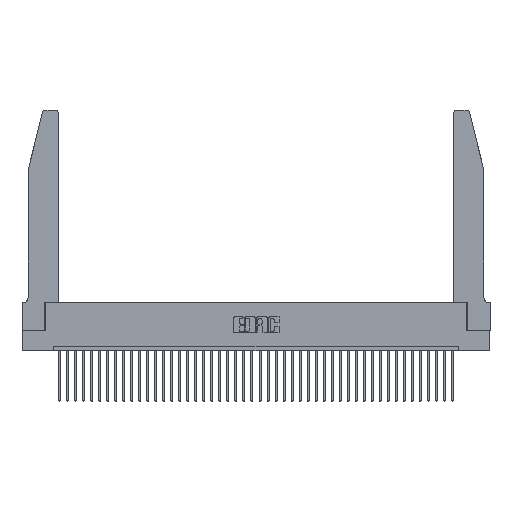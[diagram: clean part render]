
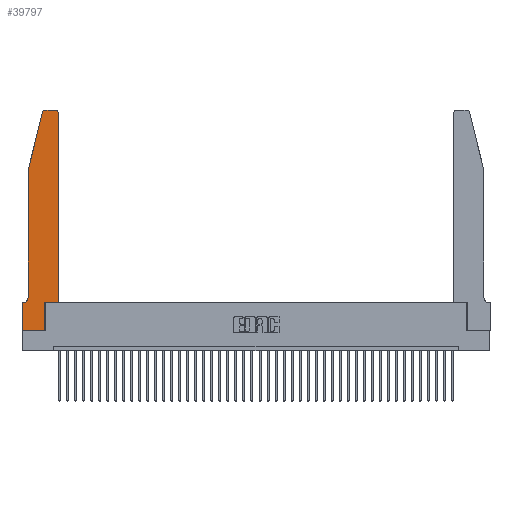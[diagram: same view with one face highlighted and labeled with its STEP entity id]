
A CAD part, top view. The second image highlights one B-rep face of the part: STEP entity #39797.
In plain terms, the highlighted planar face has unit normal (0, 0, 1).
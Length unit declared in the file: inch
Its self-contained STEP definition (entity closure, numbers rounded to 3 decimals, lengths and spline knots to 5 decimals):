
#245 = CARTESIAN_POINT ( 'NONE',  ( 0.2605, 2.75, 0.37 ) ) ;
#407 = DIRECTION ( 'NONE',  ( 0., 0., 1. ) ) ;
#1341 = EDGE_CURVE ( 'NONE', #6406, #1973, #36287, .T. ) ;
#1725 = ORIENTED_EDGE ( 'NONE', *, *, #28265, .T. ) ;
#1838 = CARTESIAN_POINT ( 'NONE',  ( 0.0755, 0.42, 0.37 ) ) ;
#1933 = VECTOR ( 'NONE', #41183, 39.37008 ) ;
#1973 = VERTEX_POINT ( 'NONE', #23858 ) ;
#3191 = VECTOR ( 'NONE', #6481, 39.37008 ) ;
#3298 = EDGE_CURVE ( 'NONE', #7035, #13448, #33613, .T. ) ;
#3389 = CIRCLE ( 'NONE', #29371, 0.07 ) ;
#3445 = DIRECTION ( 'NONE',  ( 0., -1., 0. ) ) ;
#4053 = VECTOR ( 'NONE', #23248, 39.37008 ) ;
#4185 = EDGE_CURVE ( 'NONE', #31133, #15179, #14031, .T. ) ;
#4513 = ORIENTED_EDGE ( 'NONE', *, *, #4185, .T. ) ;
#4682 = AXIS2_PLACEMENT_3D ( 'NONE', #6914, #13585, #29245 ) ;
#5447 = CARTESIAN_POINT ( 'NONE',  ( 0., 0., 0.37 ) ) ;
#5578 = EDGE_CURVE ( 'NONE', #13024, #22417, #24457, .T. ) ;
#5705 = CARTESIAN_POINT ( 'NONE',  ( 0.2865, 0.35, 0.37 ) ) ;
#5996 = CARTESIAN_POINT ( 'NONE',  ( 0.4205, 2.72, 0.37 ) ) ;
#6406 = VERTEX_POINT ( 'NONE', #21333 ) ;
#6481 = DIRECTION ( 'NONE',  ( -1., 0., 0. ) ) ;
#6540 = DIRECTION ( 'NONE',  ( 0., 1., 0. ) ) ;
#6914 = CARTESIAN_POINT ( 'NONE',  ( 0.284, 2.72, 0.37 ) ) ;
#7035 = VERTEX_POINT ( 'NONE', #37750 ) ;
#8362 = EDGE_CURVE ( 'NONE', #13448, #25497, #3389, .T. ) ;
#9171 = DIRECTION ( 'NONE',  ( 1., 0., 0. ) ) ;
#9364 = ORIENTED_EDGE ( 'NONE', *, *, #33324, .T. ) ;
#10169 = AXIS2_PLACEMENT_3D ( 'NONE', #5996, #28294, #9171 ) ;
#10204 = VECTOR ( 'NONE', #11712, 39.37008 ) ;
#10423 = VECTOR ( 'NONE', #3445, 39.37008 ) ;
#11712 = DIRECTION ( 'NONE',  ( -1., 0., 0. ) ) ;
#11817 = AXIS2_PLACEMENT_3D ( 'NONE', #38671, #407, #22762 ) ;
#12110 = LINE ( 'NONE', #245, #3191 ) ;
#12768 = ORIENTED_EDGE ( 'NONE', *, *, #27010, .T. ) ;
#13024 = VERTEX_POINT ( 'NONE', #29692 ) ;
#13448 = VERTEX_POINT ( 'NONE', #1838 ) ;
#13585 = DIRECTION ( 'NONE',  ( 0., 0., 1. ) ) ;
#13848 = ORIENTED_EDGE ( 'NONE', *, *, #37154, .T. ) ;
#13956 = LINE ( 'NONE', #5705, #36437 ) ;
#14031 = CIRCLE ( 'NONE', #4682, 0.03 ) ;
#15179 = VERTEX_POINT ( 'NONE', #17177 ) ;
#16209 = ORIENTED_EDGE ( 'NONE', *, *, #40205, .T. ) ;
#16893 = CIRCLE ( 'NONE', #10169, 0.03 ) ;
#17177 = CARTESIAN_POINT ( 'NONE',  ( 0.25487, 2.72718, 0.37 ) ) ;
#17616 = DIRECTION ( 'NONE',  ( 0., 0., -1. ) ) ;
#17843 = VERTEX_POINT ( 'NONE', #24147 ) ;
#17904 = ORIENTED_EDGE ( 'NONE', *, *, #8362, .T. ) ;
#18003 = DIRECTION ( 'NONE',  ( 0., -1., 0. ) ) ;
#19021 = CARTESIAN_POINT ( 'NONE',  ( 0.284, 2.75, 0.37 ) ) ;
#19535 = VECTOR ( 'NONE', #37322, 39.37008 ) ;
#19695 = PLANE ( 'NONE',  #11817 ) ;
#20122 = VERTEX_POINT ( 'NONE', #32387 ) ;
#20123 = CARTESIAN_POINT ( 'NONE',  ( 0., 0., 0.37 ) ) ;
#20538 = ORIENTED_EDGE ( 'NONE', *, *, #3298, .T. ) ;
#21333 = CARTESIAN_POINT ( 'NONE',  ( 0.4505, 0.35, 0.37 ) ) ;
#22417 = VERTEX_POINT ( 'NONE', #20123 ) ;
#22493 = LINE ( 'NONE', #26629, #4053 ) ;
#22693 = ORIENTED_EDGE ( 'NONE', *, *, #27812, .T. ) ;
#22762 = DIRECTION ( 'NONE',  ( 1., 0., 0. ) ) ;
#23248 = DIRECTION ( 'NONE',  ( -0.239, -0.971, 0. ) ) ;
#23458 = CARTESIAN_POINT ( 'NONE',  ( 0.4205, 2.75, 0.37 ) ) ;
#23858 = CARTESIAN_POINT ( 'NONE',  ( 0.4505, 2.72, 0.37 ) ) ;
#24147 = CARTESIAN_POINT ( 'NONE',  ( 0.2865, 0.35, 0.37 ) ) ;
#24457 = LINE ( 'NONE', #27457, #10423 ) ;
#25163 = CARTESIAN_POINT ( 'NONE',  ( 0.4505, 0.35, 0.37 ) ) ;
#25245 = LINE ( 'NONE', #27810, #10204 ) ;
#25372 = ORIENTED_EDGE ( 'NONE', *, *, #5578, .T. ) ;
#25497 = VERTEX_POINT ( 'NONE', #40124 ) ;
#25912 = CARTESIAN_POINT ( 'NONE',  ( 0.4505, 0.35, 0.37 ) ) ;
#26322 = LINE ( 'NONE', #25163, #1933 ) ;
#26629 = CARTESIAN_POINT ( 'NONE',  ( 0.0755, 2., 0.37 ) ) ;
#26848 = VECTOR ( 'NONE', #39553, 39.37008 ) ;
#27010 = EDGE_CURVE ( 'NONE', #22417, #20122, #40565, .T. ) ;
#27457 = CARTESIAN_POINT ( 'NONE',  ( 0., 0., 0.37 ) ) ;
#27810 = CARTESIAN_POINT ( 'NONE',  ( 0.0755, 0.35, 0.37 ) ) ;
#27812 = EDGE_CURVE ( 'NONE', #15179, #7035, #22493, .T. ) ;
#28265 = EDGE_CURVE ( 'NONE', #20122, #17843, #13956, .T. ) ;
#28294 = DIRECTION ( 'NONE',  ( 0., 0., 1. ) ) ;
#28799 = EDGE_CURVE ( 'NONE', #1973, #30607, #16893, .T. ) ;
#29245 = DIRECTION ( 'NONE',  ( 1., 0., 0. ) ) ;
#29371 = AXIS2_PLACEMENT_3D ( 'NONE', #33347, #17616, #39927 ) ;
#29692 = CARTESIAN_POINT ( 'NONE',  ( 0., 0.35, 0.37 ) ) ;
#30607 = VERTEX_POINT ( 'NONE', #23458 ) ;
#31133 = VERTEX_POINT ( 'NONE', #19021 ) ;
#31264 = CARTESIAN_POINT ( 'NONE',  ( 0.0755, 2., 0.37 ) ) ;
#32387 = CARTESIAN_POINT ( 'NONE',  ( 0.2865, 0., 0.37 ) ) ;
#33324 = EDGE_CURVE ( 'NONE', #30607, #31133, #12110, .T. ) ;
#33347 = CARTESIAN_POINT ( 'NONE',  ( 0.0055, 0.42, 0.37 ) ) ;
#33613 = LINE ( 'NONE', #31264, #38139 ) ;
#36287 = LINE ( 'NONE', #25912, #26848 ) ;
#36437 = VECTOR ( 'NONE', #6540, 39.37008 ) ;
#37154 = EDGE_CURVE ( 'NONE', #17843, #6406, #26322, .T. ) ;
#37322 = DIRECTION ( 'NONE',  ( 1., 0., 0. ) ) ;
#37750 = CARTESIAN_POINT ( 'NONE',  ( 0.0755, 2., 0.37 ) ) ;
#38061 = ORIENTED_EDGE ( 'NONE', *, *, #1341, .T. ) ;
#38139 = VECTOR ( 'NONE', #18003, 39.37008 ) ;
#38357 = EDGE_LOOP ( 'NONE', ( #9364, #4513, #22693, #20538, #17904, #16209, #25372, #12768, #1725, #13848, #38061, #38789 ) ) ;
#38671 = CARTESIAN_POINT ( 'NONE',  ( 0., 0.35, 0.37 ) ) ;
#38789 = ORIENTED_EDGE ( 'NONE', *, *, #28799, .T. ) ;
#39553 = DIRECTION ( 'NONE',  ( 0., 1., 0. ) ) ;
#39718 = FACE_OUTER_BOUND ( 'NONE', #38357, .T. ) ;
#39797 = ADVANCED_FACE ( 'NONE', ( #39718 ), #19695, .T. ) ;
#39927 = DIRECTION ( 'NONE',  ( -1., 0., 0. ) ) ;
#40124 = CARTESIAN_POINT ( 'NONE',  ( 0.0055, 0.35, 0.37 ) ) ;
#40205 = EDGE_CURVE ( 'NONE', #25497, #13024, #25245, .T. ) ;
#40565 = LINE ( 'NONE', #5447, #19535 ) ;
#41183 = DIRECTION ( 'NONE',  ( 1., 0., 0. ) ) ;
